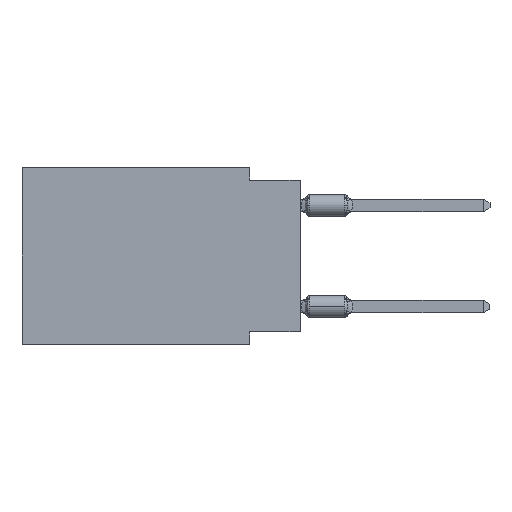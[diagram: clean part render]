
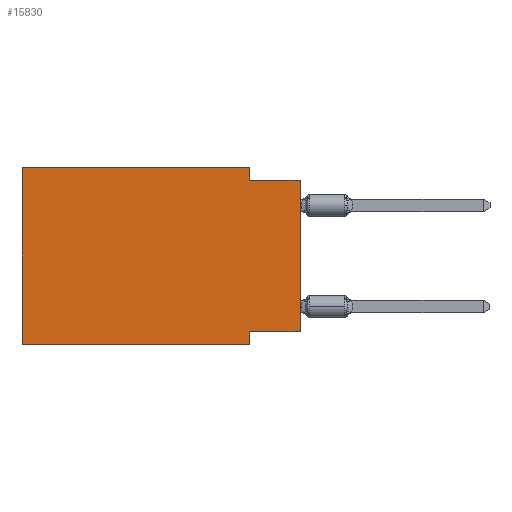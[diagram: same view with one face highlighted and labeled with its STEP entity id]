
A CAD part, left-side view. The second image highlights one B-rep face of the part: STEP entity #15830.
In plain terms, the highlighted planar face has unit normal (-1, 0, 0).
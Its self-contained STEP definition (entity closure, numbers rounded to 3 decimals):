
#743 = CARTESIAN_POINT ( 'NONE',  ( 0., 13.97, 0. ) ) ;
#1275 = EDGE_LOOP ( 'NONE', ( #19520, #6625, #11025, #12767, #4072, #4118, #6766, #2995 ) ) ;
#1561 = DIRECTION ( 'NONE',  ( 1., 0., 0. ) ) ;
#1911 = EDGE_CURVE ( 'NONE', #10842, #9843, #3873, .T. ) ;
#2135 = DIRECTION ( 'NONE',  ( 0., 0., -1. ) ) ;
#2262 = CARTESIAN_POINT ( 'NONE',  ( 0., 13.97, 0. ) ) ;
#2513 = CARTESIAN_POINT ( 'NONE',  ( 0., 0., 0. ) ) ;
#2995 = ORIENTED_EDGE ( 'NONE', *, *, #4218, .F. ) ;
#3873 = LINE ( 'NONE', #13630, #11944 ) ;
#4072 = ORIENTED_EDGE ( 'NONE', *, *, #10514, .F. ) ;
#4118 = ORIENTED_EDGE ( 'NONE', *, *, #1911, .T. ) ;
#4218 = EDGE_CURVE ( 'NONE', #4790, #15182, #8610, .T. ) ;
#4790 = VERTEX_POINT ( 'NONE', #20458 ) ;
#4810 = EDGE_CURVE ( 'NONE', #17954, #10658, #10602, .T. ) ;
#5209 = EDGE_CURVE ( 'NONE', #9466, #10351, #9178, .T. ) ;
#5317 = CARTESIAN_POINT ( 'NONE',  ( 0., 2.54, -8.89 ) ) ;
#5653 = EDGE_CURVE ( 'NONE', #4790, #10351, #18892, .T. ) ;
#6072 = VECTOR ( 'NONE', #7901, 1000. ) ;
#6279 = DIRECTION ( 'NONE',  ( 0., 0., -1. ) ) ;
#6625 = ORIENTED_EDGE ( 'NONE', *, *, #5209, .F. ) ;
#6632 = VECTOR ( 'NONE', #19240, 1000. ) ;
#6766 = ORIENTED_EDGE ( 'NONE', *, *, #13079, .F. ) ;
#6881 = VECTOR ( 'NONE', #18627, 1000. ) ;
#6995 = CARTESIAN_POINT ( 'NONE',  ( 0., 0., -8.255 ) ) ;
#7763 = DIRECTION ( 'NONE',  ( 0., 0., 1. ) ) ;
#7901 = DIRECTION ( 'NONE',  ( 0., 1., 0. ) ) ;
#8003 = CARTESIAN_POINT ( 'NONE',  ( 0., 0., -0.635 ) ) ;
#8088 = AXIS2_PLACEMENT_3D ( 'NONE', #8205, #1561, #6279 ) ;
#8089 = EDGE_CURVE ( 'NONE', #10658, #9466, #19905, .T. ) ;
#8179 = CARTESIAN_POINT ( 'NONE',  ( 0., 2.54, -8.255 ) ) ;
#8205 = CARTESIAN_POINT ( 'NONE',  ( 0., 13.97, 0. ) ) ;
#8610 = LINE ( 'NONE', #6995, #6072 ) ;
#9178 = LINE ( 'NONE', #8003, #6632 ) ;
#9466 = VERTEX_POINT ( 'NONE', #17648 ) ;
#9843 = VERTEX_POINT ( 'NONE', #10997 ) ;
#10351 = VERTEX_POINT ( 'NONE', #15999 ) ;
#10403 = VECTOR ( 'NONE', #7763, 1000. ) ;
#10434 = VECTOR ( 'NONE', #2135, 1000. ) ;
#10514 = EDGE_CURVE ( 'NONE', #10842, #17954, #19747, .T. ) ;
#10602 = LINE ( 'NONE', #743, #10863 ) ;
#10658 = VERTEX_POINT ( 'NONE', #20891 ) ;
#10842 = VERTEX_POINT ( 'NONE', #13382 ) ;
#10863 = VECTOR ( 'NONE', #18411, 1000. ) ;
#10997 = CARTESIAN_POINT ( 'NONE',  ( 0., 2.54, -8.89 ) ) ;
#11025 = ORIENTED_EDGE ( 'NONE', *, *, #8089, .F. ) ;
#11208 = PLANE ( 'NONE',  #8088 ) ;
#11670 = CARTESIAN_POINT ( 'NONE',  ( 0., 2.54, 0. ) ) ;
#11944 = VECTOR ( 'NONE', #15329, 1000. ) ;
#12767 = ORIENTED_EDGE ( 'NONE', *, *, #4810, .F. ) ;
#13079 = EDGE_CURVE ( 'NONE', #15182, #9843, #19777, .T. ) ;
#13382 = CARTESIAN_POINT ( 'NONE',  ( 0., 13.97, -8.89 ) ) ;
#13630 = CARTESIAN_POINT ( 'NONE',  ( 0., 13.97, -8.89 ) ) ;
#15182 = VERTEX_POINT ( 'NONE', #8179 ) ;
#15329 = DIRECTION ( 'NONE',  ( 0., -1., 0. ) ) ;
#15830 = ADVANCED_FACE ( 'NONE', ( #19334 ), #11208, .F. ) ;
#15999 = CARTESIAN_POINT ( 'NONE',  ( 0., 0., -0.635 ) ) ;
#17228 = CARTESIAN_POINT ( 'NONE',  ( 0., 13.97, 0. ) ) ;
#17648 = CARTESIAN_POINT ( 'NONE',  ( 0., 2.54, -0.635 ) ) ;
#17954 = VERTEX_POINT ( 'NONE', #17228 ) ;
#18261 = DIRECTION ( 'NONE',  ( 0., 0., -1. ) ) ;
#18411 = DIRECTION ( 'NONE',  ( 0., -1., 0. ) ) ;
#18627 = DIRECTION ( 'NONE',  ( 0., 0., 1. ) ) ;
#18892 = LINE ( 'NONE', #2513, #10403 ) ;
#19061 = VECTOR ( 'NONE', #18261, 1000. ) ;
#19240 = DIRECTION ( 'NONE',  ( 0., -1., 0. ) ) ;
#19334 = FACE_OUTER_BOUND ( 'NONE', #1275, .T. ) ;
#19520 = ORIENTED_EDGE ( 'NONE', *, *, #5653, .T. ) ;
#19747 = LINE ( 'NONE', #2262, #6881 ) ;
#19777 = LINE ( 'NONE', #5317, #19061 ) ;
#19905 = LINE ( 'NONE', #11670, #10434 ) ;
#20458 = CARTESIAN_POINT ( 'NONE',  ( 0., 0., -8.255 ) ) ;
#20891 = CARTESIAN_POINT ( 'NONE',  ( 0., 2.54, 0. ) ) ;
